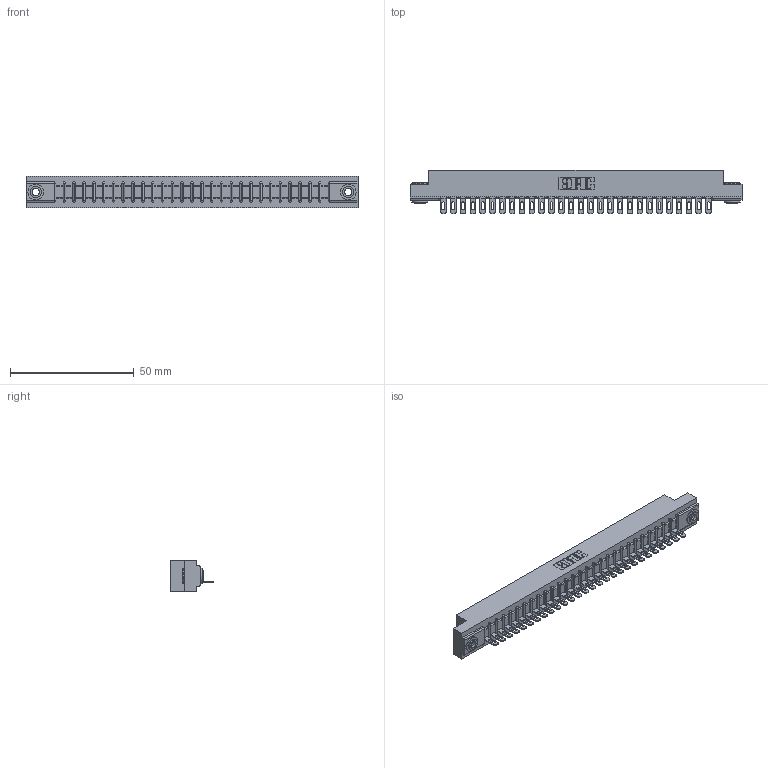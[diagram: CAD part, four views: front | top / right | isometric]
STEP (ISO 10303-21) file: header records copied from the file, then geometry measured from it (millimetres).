
FILE_DESCRIPTION (( 'STEP AP203' ), '1' );
FILE_NAME ('307-028-501-103.STEP', '2018-08-04T16:14:27', ( '' ), ( '' ), 'SwSTEP 2.0', 'SolidWorks 2016', '' );
FILE_SCHEMA (( 'CONFIG_CONTROL_DESIGN' ));
Length unit declared in the file: inch
Products named in the file (4): 307-028-501-103; 307 Part_.156 Dia Mounting Holes; 307-290-002_501; 345-250-002_345-250-002-102
Assembly tree (31 placements, depth 2):
  307-028-501-103
    307 Part_.156 Dia Mounting Holes
    307-290-002_501  x28
    345-250-002_345-250-002-102  x2
Bounding box: 133.96 x 17.42 x 12.7 mm (x, y, z)
Volume: 14256.7 mm3; surface area: 18057.7 mm2
Topology: 31 solids, 31 shells, 2327 faces, 7099 edges, 4650 vertices
Faces by surface type: plane 1326, cylinder 935, sphere 58, cone 8
Entity records: 27589 total; most frequent: CARTESIAN_POINT 4629, ORIENTED_EDGE 4610, DIRECTION 4523, EDGE_CURVE 2305, LINE 1747, VECTOR 1747, VERTEX_POINT 1494, AXIS2_PLACEMENT_3D 1388
